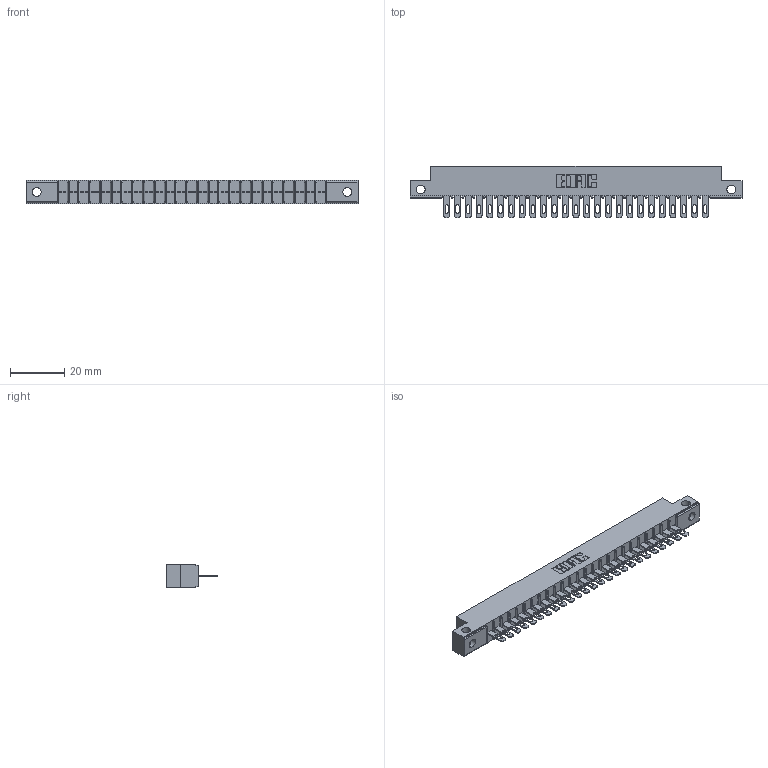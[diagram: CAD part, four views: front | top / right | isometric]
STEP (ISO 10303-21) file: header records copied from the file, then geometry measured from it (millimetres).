
FILE_DESCRIPTION (( 'STEP AP203' ), '1' );
FILE_NAME ('316-025-400-112.STEP', '2020-09-22T21:50:02', ( '' ), ( '' ), 'SwSTEP 2.0', 'SolidWorks 2020', '' );
FILE_SCHEMA (( 'CONFIG_CONTROL_DESIGN' ));
Length unit declared in the file: inch
Products named in the file (3): 306 Part_.128 Dia; 306-290-001_100; 316-025-400-112
Assembly tree (26 placements, depth 2):
  316-025-400-112
    306 Part_.128 Dia
    306-290-001_100  x25
Bounding box: 122.07 x 18.87 x 8.71 mm (x, y, z)
Volume: 8310.9 mm3; surface area: 12715.7 mm2
Topology: 26 solids, 26 shells, 2028 faces, 5727 edges, 3678 vertices
Faces by surface type: plane 1318, cylinder 610, sphere 100
Entity records: 26086 total; most frequent: CARTESIAN_POINT 4426, ORIENTED_EDGE 4342, DIRECTION 4305, EDGE_CURVE 2171, VECTOR 1671, LINE 1671, VERTEX_POINT 1374, AXIS2_PLACEMENT_3D 1317
